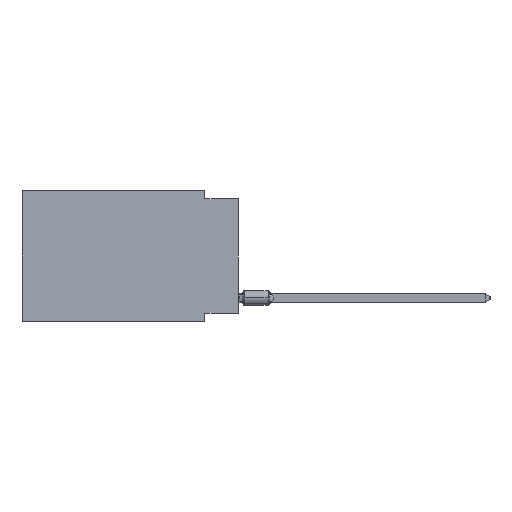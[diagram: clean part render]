
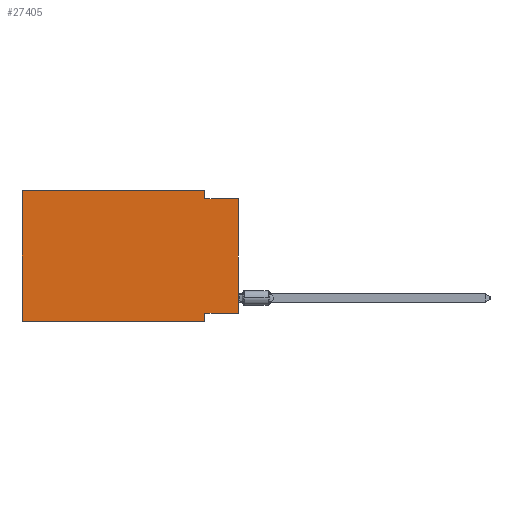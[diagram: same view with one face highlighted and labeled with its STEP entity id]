
A CAD part, left-side view. The second image highlights one B-rep face of the part: STEP entity #27405.
In plain terms, the highlighted planar face has unit normal (-1, 0, 0).
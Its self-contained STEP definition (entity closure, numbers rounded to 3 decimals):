
#313 = EDGE_CURVE ( 'NONE', #30855, #46329, #52064, .T. ) ;
#1050 = ORIENTED_EDGE ( 'NONE', *, *, #2689, .F. ) ;
#2165 = ORIENTED_EDGE ( 'NONE', *, *, #55266, .T. ) ;
#2689 = EDGE_CURVE ( 'NONE', #42566, #67697, #21056, .T. ) ;
#6049 = DIRECTION ( 'NONE',  ( 0., 0., -1. ) ) ;
#6169 = CARTESIAN_POINT ( 'NONE',  ( 0., 0., -0.635 ) ) ;
#7306 = CARTESIAN_POINT ( 'NONE',  ( 0., 0., 0. ) ) ;
#9020 = VECTOR ( 'NONE', #16081, 1000. ) ;
#9125 = LINE ( 'NONE', #31057, #65186 ) ;
#10850 = EDGE_CURVE ( 'NONE', #37393, #33403, #59155, .T. ) ;
#11298 = CARTESIAN_POINT ( 'NONE',  ( 0., 2.54, -9.906 ) ) ;
#13152 = ORIENTED_EDGE ( 'NONE', *, *, #27721, .F. ) ;
#13183 = ORIENTED_EDGE ( 'NONE', *, *, #60853, .T. ) ;
#13641 = CARTESIAN_POINT ( 'NONE',  ( 0., 0., -0.635 ) ) ;
#14110 = DIRECTION ( 'NONE',  ( 1., 0., 0. ) ) ;
#16081 = DIRECTION ( 'NONE',  ( 0., 0., 1. ) ) ;
#16940 = VECTOR ( 'NONE', #30134, 1000. ) ;
#17754 = LINE ( 'NONE', #7306, #23367 ) ;
#18654 = PLANE ( 'NONE',  #51328 ) ;
#20008 = VECTOR ( 'NONE', #64374, 1000. ) ;
#21056 = LINE ( 'NONE', #11298, #22618 ) ;
#22618 = VECTOR ( 'NONE', #32575, 1000. ) ;
#23367 = VECTOR ( 'NONE', #64833, 1000. ) ;
#26681 = CARTESIAN_POINT ( 'NONE',  ( 0., 16.383, -9.906 ) ) ;
#27405 = ADVANCED_FACE ( 'NONE', ( #29469 ), #18654, .F. ) ;
#27721 = EDGE_CURVE ( 'NONE', #46329, #37393, #49621, .T. ) ;
#28181 = ORIENTED_EDGE ( 'NONE', *, *, #41139, .F. ) ;
#28362 = CARTESIAN_POINT ( 'NONE',  ( 0., 2.54, 0. ) ) ;
#29469 = FACE_OUTER_BOUND ( 'NONE', #42940, .T. ) ;
#30134 = DIRECTION ( 'NONE',  ( 0., -1., 0. ) ) ;
#30855 = VERTEX_POINT ( 'NONE', #48945 ) ;
#31057 = CARTESIAN_POINT ( 'NONE',  ( 0., 16.383, -9.906 ) ) ;
#32121 = ORIENTED_EDGE ( 'NONE', *, *, #10850, .F. ) ;
#32575 = DIRECTION ( 'NONE',  ( 0., 0., -1. ) ) ;
#33403 = VERTEX_POINT ( 'NONE', #13641 ) ;
#35046 = CARTESIAN_POINT ( 'NONE',  ( 0., 16.383, 0. ) ) ;
#35977 = DIRECTION ( 'NONE',  ( 0., 1., 0. ) ) ;
#37393 = VERTEX_POINT ( 'NONE', #52765 ) ;
#37519 = CARTESIAN_POINT ( 'NONE',  ( 0., 2.54, -9.906 ) ) ;
#39509 = CARTESIAN_POINT ( 'NONE',  ( 0., 0., -9.271 ) ) ;
#40884 = VERTEX_POINT ( 'NONE', #39509 ) ;
#41139 = EDGE_CURVE ( 'NONE', #49331, #30855, #53368, .T. ) ;
#41267 = CARTESIAN_POINT ( 'NONE',  ( 0., 16.383, 0. ) ) ;
#41876 = CARTESIAN_POINT ( 'NONE',  ( 0., 0., -9.271 ) ) ;
#42566 = VERTEX_POINT ( 'NONE', #50928 ) ;
#42663 = CARTESIAN_POINT ( 'NONE',  ( 0., 2.54, 0. ) ) ;
#42940 = EDGE_LOOP ( 'NONE', ( #13183, #32121, #13152, #66957, #28181, #2165, #1050, #58889 ) ) ;
#44263 = EDGE_CURVE ( 'NONE', #40884, #42566, #63131, .T. ) ;
#46329 = VERTEX_POINT ( 'NONE', #42663 ) ;
#48286 = VECTOR ( 'NONE', #35977, 1000. ) ;
#48945 = CARTESIAN_POINT ( 'NONE',  ( 0., 16.383, 0. ) ) ;
#49331 = VERTEX_POINT ( 'NONE', #26681 ) ;
#49621 = LINE ( 'NONE', #28362, #59094 ) ;
#50928 = CARTESIAN_POINT ( 'NONE',  ( 0., 2.54, -9.271 ) ) ;
#51328 = AXIS2_PLACEMENT_3D ( 'NONE', #35046, #14110, #67756 ) ;
#52064 = LINE ( 'NONE', #41267, #16940 ) ;
#52765 = CARTESIAN_POINT ( 'NONE',  ( 0., 2.54, -0.635 ) ) ;
#53368 = LINE ( 'NONE', #63838, #9020 ) ;
#55266 = EDGE_CURVE ( 'NONE', #49331, #67697, #9125, .T. ) ;
#57553 = DIRECTION ( 'NONE',  ( 0., -1., 0. ) ) ;
#58889 = ORIENTED_EDGE ( 'NONE', *, *, #44263, .F. ) ;
#59094 = VECTOR ( 'NONE', #6049, 1000. ) ;
#59155 = LINE ( 'NONE', #6169, #20008 ) ;
#60853 = EDGE_CURVE ( 'NONE', #40884, #33403, #17754, .T. ) ;
#63131 = LINE ( 'NONE', #41876, #48286 ) ;
#63838 = CARTESIAN_POINT ( 'NONE',  ( 0., 16.383, 0. ) ) ;
#64374 = DIRECTION ( 'NONE',  ( 0., -1., 0. ) ) ;
#64833 = DIRECTION ( 'NONE',  ( 0., 0., 1. ) ) ;
#65186 = VECTOR ( 'NONE', #57553, 1000. ) ;
#66957 = ORIENTED_EDGE ( 'NONE', *, *, #313, .F. ) ;
#67697 = VERTEX_POINT ( 'NONE', #37519 ) ;
#67756 = DIRECTION ( 'NONE',  ( 0., 0., -1. ) ) ;
